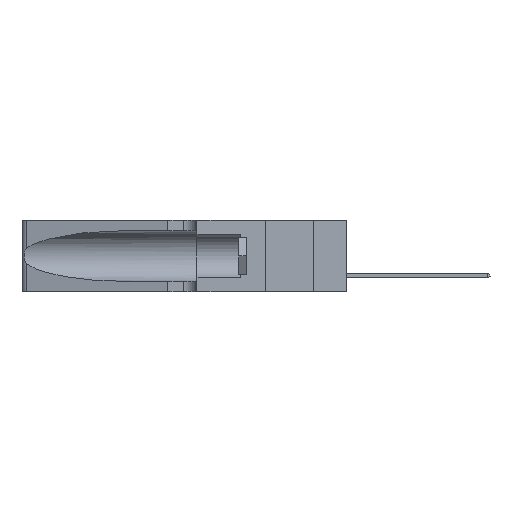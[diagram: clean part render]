
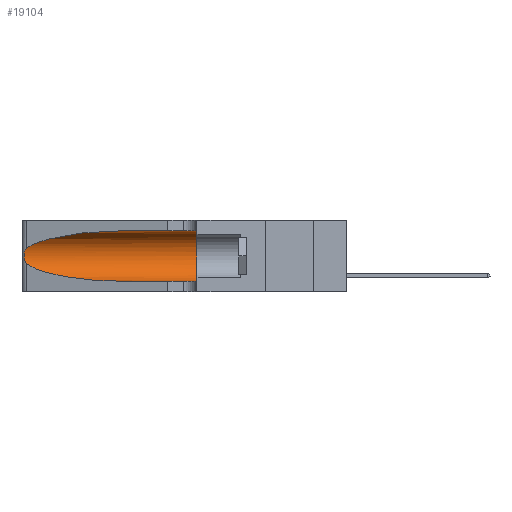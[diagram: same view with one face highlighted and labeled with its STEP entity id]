
A CAD part, left-side view. The second image highlights one B-rep face of the part: STEP entity #19104.
In plain terms, the highlighted cylindrical face has radius 3.308 mm (diameter 6.617 mm), a partial arc.
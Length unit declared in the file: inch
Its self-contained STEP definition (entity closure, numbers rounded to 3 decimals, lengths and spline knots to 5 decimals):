
#386 =( BOUNDED_CURVE ( )  B_SPLINE_CURVE ( 3, ( #19266, #745, #19691, #25793 ),
 .UNSPECIFIED., .F., .T. ) 
 B_SPLINE_CURVE_WITH_KNOTS ( ( 4, 4 ),
 ( 3.44316, 4.71239 ),
 .UNSPECIFIED. ) 
 CURVE ( )  GEOMETRIC_REPRESENTATION_ITEM ( )  RATIONAL_B_SPLINE_CURVE ( ( 1., 0.87, 0.87, 1. ) ) 
 REPRESENTATION_ITEM ( '' )  );
#745 = CARTESIAN_POINT ( 'NONE',  ( 0.2373, 1.15595, 0.08982 ) ) ;
#1556 = CARTESIAN_POINT ( 'NONE',  ( 0.25639, 1.23184, 0.21858 ) ) ;
#2194 = CYLINDRICAL_SURFACE ( 'NONE', #32175, 0.13025 ) ;
#2241 = CARTESIAN_POINT ( 'NONE',  ( 0.1305, 0.72297, 0.31525 ) ) ;
#3368 = CARTESIAN_POINT ( 'NONE',  ( 0.1305, 1.61858, 0.31525 ) ) ;
#3424 = EDGE_CURVE ( 'NONE', #36043, #30346, #386, .T. ) ;
#3954 = CARTESIAN_POINT ( 'NONE',  ( 0.1305, 0.35, 0.185 ) ) ;
#4122 = CARTESIAN_POINT ( 'NONE',  ( 0.1305, 0.72297, 0.31525 ) ) ;
#4165 = ORIENTED_EDGE ( 'NONE', *, *, #7638, .T. ) ;
#4801 = CARTESIAN_POINT ( 'NONE',  ( 0.25487, 1.22718, 0.22369 ) ) ;
#5490 = CARTESIAN_POINT ( 'NONE',  ( 0.1305, 1.61858, 0.185 ) ) ;
#6286 = VERTEX_POINT ( 'NONE', #2241 ) ;
#7638 = EDGE_CURVE ( 'NONE', #6286, #30152, #30448, .T. ) ;
#7867 = CARTESIAN_POINT ( 'NONE',  ( 0.25856, 1.23593, 0.16098 ) ) ;
#9763 = B_SPLINE_CURVE_WITH_KNOTS ( 'NONE', 3,
 ( #4801, #13692, #1556, #26059, #14097, #19975, #23497, #20113, #26466, #7867, #29604, #35812, #17228, #20380 ),
 .UNSPECIFIED., .F., .F.,
 ( 4, 2, 2, 2, 2, 2, 4 ),
 ( 0., 0.00027, 0.00053, 0.00107, 0.0016, 0.00187, 0.00214 ),
 .UNSPECIFIED. ) ;
#11800 = FACE_OUTER_BOUND ( 'NONE', #28906, .T. ) ;
#12290 = ORIENTED_EDGE ( 'NONE', *, *, #14766, .T. ) ;
#12419 = CARTESIAN_POINT ( 'NONE',  ( 0.1305, 0.35, 0.05475 ) ) ;
#13220 = VERTEX_POINT ( 'NONE', #12419 ) ;
#13692 = CARTESIAN_POINT ( 'NONE',  ( 0.25555, 1.22994, 0.2215 ) ) ;
#14097 = CARTESIAN_POINT ( 'NONE',  ( 0.25854, 1.2359, 0.20912 ) ) ;
#14766 = EDGE_CURVE ( 'NONE', #30346, #13220, #20573, .T. ) ;
#15894 = VECTOR ( 'NONE', #21938, 39.37008 ) ;
#16518 = CARTESIAN_POINT ( 'NONE',  ( 0.25487, 1.22718, 0.22369 ) ) ;
#16806 = DIRECTION ( 'NONE',  ( 0., 1., 0. ) ) ;
#16853 = CARTESIAN_POINT ( 'NONE',  ( 0.1305, 1.61858, 0.05475 ) ) ;
#17228 = CARTESIAN_POINT ( 'NONE',  ( 0.25555, 1.22993, 0.14849 ) ) ;
#17806 = EDGE_CURVE ( 'NONE', #21615, #13220, #21168, .T. ) ;
#19104 = ADVANCED_FACE ( 'NONE', ( #11800 ), #2194, .F. ) ;
#19266 = CARTESIAN_POINT ( 'NONE',  ( 0.25487, 1.22718, 0.14631 ) ) ;
#19691 = CARTESIAN_POINT ( 'NONE',  ( 0.18966, 0.96281, 0.05475 ) ) ;
#19954 = EDGE_CURVE ( 'NONE', #30152, #36043, #9763, .T. ) ;
#19975 = CARTESIAN_POINT ( 'NONE',  ( 0.26018, 1.23835, 0.19895 ) ) ;
#20113 = CARTESIAN_POINT ( 'NONE',  ( 0.26075, 1.23896, 0.178 ) ) ;
#20380 = CARTESIAN_POINT ( 'NONE',  ( 0.25487, 1.22718, 0.14631 ) ) ;
#20573 = LINE ( 'NONE', #16853, #39941 ) ;
#21168 = CIRCLE ( 'NONE', #22814, 0.13025 ) ;
#21615 = VERTEX_POINT ( 'NONE', #31506 ) ;
#21938 = DIRECTION ( 'NONE',  ( 0., -1., 0. ) ) ;
#22143 = ORIENTED_EDGE ( 'NONE', *, *, #3424, .T. ) ;
#22486 = EDGE_CURVE ( 'NONE', #6286, #21615, #38226, .T. ) ;
#22814 = AXIS2_PLACEMENT_3D ( 'NONE', #3954, #16806, #35121 ) ;
#23497 = CARTESIAN_POINT ( 'NONE',  ( 0.26075, 1.23896, 0.19203 ) ) ;
#25368 = CARTESIAN_POINT ( 'NONE',  ( 0.2373, 1.15595, 0.28018 ) ) ;
#25793 = CARTESIAN_POINT ( 'NONE',  ( 0.1305, 0.72297, 0.05475 ) ) ;
#26059 = CARTESIAN_POINT ( 'NONE',  ( 0.25787, 1.23484, 0.2124 ) ) ;
#26466 = CARTESIAN_POINT ( 'NONE',  ( 0.26017, 1.23833, 0.17102 ) ) ;
#26735 = ORIENTED_EDGE ( 'NONE', *, *, #17806, .F. ) ;
#26855 = ORIENTED_EDGE ( 'NONE', *, *, #22486, .F. ) ;
#28031 = CARTESIAN_POINT ( 'NONE',  ( 0.25487, 1.22718, 0.22369 ) ) ;
#28906 = EDGE_LOOP ( 'NONE', ( #4165, #38679, #22143, #12290, #26735, #26855 ) ) ;
#29604 = CARTESIAN_POINT ( 'NONE',  ( 0.25789, 1.23486, 0.15765 ) ) ;
#30152 = VERTEX_POINT ( 'NONE', #28031 ) ;
#30346 = VERTEX_POINT ( 'NONE', #33709 ) ;
#30385 = CARTESIAN_POINT ( 'NONE',  ( 0.25487, 1.22718, 0.14631 ) ) ;
#30429 = DIRECTION ( 'NONE',  ( 0., -1., 0. ) ) ;
#30448 =( BOUNDED_CURVE ( )  B_SPLINE_CURVE ( 3, ( #4122, #31738, #25368, #16518 ),
 .UNSPECIFIED., .F., .F. ) 
 B_SPLINE_CURVE_WITH_KNOTS ( ( 4, 4 ),
 ( 1.5708, 2.84003 ),
 .UNSPECIFIED. ) 
 CURVE ( )  GEOMETRIC_REPRESENTATION_ITEM ( )  RATIONAL_B_SPLINE_CURVE ( ( 1., 0.87, 0.87, 1. ) ) 
 REPRESENTATION_ITEM ( '' )  );
#31506 = CARTESIAN_POINT ( 'NONE',  ( 0.1305, 0.35, 0.31525 ) ) ;
#31738 = CARTESIAN_POINT ( 'NONE',  ( 0.18966, 0.96281, 0.31525 ) ) ;
#32175 = AXIS2_PLACEMENT_3D ( 'NONE', #5490, #30429, #36509 ) ;
#32874 = DIRECTION ( 'NONE',  ( 0., -1., 0. ) ) ;
#33709 = CARTESIAN_POINT ( 'NONE',  ( 0.1305, 0.72297, 0.05475 ) ) ;
#35121 = DIRECTION ( 'NONE',  ( 0., 0., 1. ) ) ;
#35812 = CARTESIAN_POINT ( 'NONE',  ( 0.25639, 1.23186, 0.15144 ) ) ;
#36043 = VERTEX_POINT ( 'NONE', #30385 ) ;
#36509 = DIRECTION ( 'NONE',  ( 0., 0., -1. ) ) ;
#38226 = LINE ( 'NONE', #3368, #15894 ) ;
#38679 = ORIENTED_EDGE ( 'NONE', *, *, #19954, .T. ) ;
#39941 = VECTOR ( 'NONE', #32874, 39.37008 ) ;
